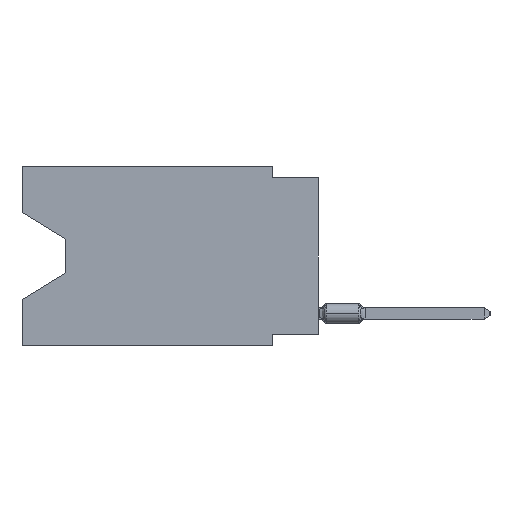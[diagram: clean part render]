
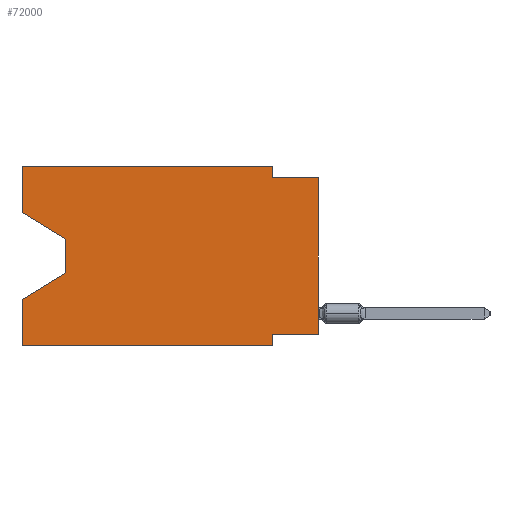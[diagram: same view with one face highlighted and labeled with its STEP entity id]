
A CAD part, left-side view. The second image highlights one B-rep face of the part: STEP entity #72000.
In plain terms, the highlighted planar face has unit normal (-1, 0, 0).
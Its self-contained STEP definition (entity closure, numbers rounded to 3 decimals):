
#440 = CARTESIAN_POINT ( 'NONE',  ( 0., 16.383, 0. ) ) ;
#507 = CARTESIAN_POINT ( 'NONE',  ( 0., 16.383, 0. ) ) ;
#642 = CARTESIAN_POINT ( 'NONE',  ( 0., 2.54, -9.906 ) ) ;
#739 = EDGE_CURVE ( 'NONE', #52487, #64820, #70216, .T. ) ;
#3649 = DIRECTION ( 'NONE',  ( 0., -1., 0. ) ) ;
#3943 = EDGE_LOOP ( 'NONE', ( #4611, #56221, #51266, #8368, #60722, #46867, #68216, #13550, #81424, #51100, #72650, #27311 ) ) ;
#4611 = ORIENTED_EDGE ( 'NONE', *, *, #12459, .T. ) ;
#5242 = CARTESIAN_POINT ( 'NONE',  ( 0., 16.383, -9.906 ) ) ;
#6098 = CARTESIAN_POINT ( 'NONE',  ( 0., 0., -9.271 ) ) ;
#8295 = EDGE_CURVE ( 'NONE', #15607, #71656, #63354, .T. ) ;
#8368 = ORIENTED_EDGE ( 'NONE', *, *, #38040, .F. ) ;
#9040 = DIRECTION ( 'NONE',  ( 0., 0., -1. ) ) ;
#9926 = CARTESIAN_POINT ( 'NONE',  ( 0., 0., -0.635 ) ) ;
#12459 = EDGE_CURVE ( 'NONE', #52487, #46699, #63314, .T. ) ;
#12963 = CARTESIAN_POINT ( 'NONE',  ( 0., 16.383, 0. ) ) ;
#13550 = ORIENTED_EDGE ( 'NONE', *, *, #52747, .T. ) ;
#13560 = DIRECTION ( 'NONE',  ( 0., -0.855, -0.519 ) ) ;
#15607 = VERTEX_POINT ( 'NONE', #53150 ) ;
#16781 = DIRECTION ( 'NONE',  ( 0., 0., -1. ) ) ;
#18680 = LINE ( 'NONE', #26591, #46604 ) ;
#19165 = VERTEX_POINT ( 'NONE', #642 ) ;
#20606 = LINE ( 'NONE', #39845, #56471 ) ;
#21585 = FACE_OUTER_BOUND ( 'NONE', #3943, .T. ) ;
#22168 = VECTOR ( 'NONE', #16781, 1000. ) ;
#22882 = EDGE_CURVE ( 'NONE', #46699, #24550, #68189, .T. ) ;
#23731 = CARTESIAN_POINT ( 'NONE',  ( 0., 16.383, -2.546 ) ) ;
#24550 = VERTEX_POINT ( 'NONE', #35504 ) ;
#24556 = DIRECTION ( 'NONE',  ( 0., 0.855, -0.519 ) ) ;
#24721 = VERTEX_POINT ( 'NONE', #5242 ) ;
#25302 = LINE ( 'NONE', #73493, #69321 ) ;
#25745 = VERTEX_POINT ( 'NONE', #40839 ) ;
#26591 = CARTESIAN_POINT ( 'NONE',  ( 0., 0., 0. ) ) ;
#27300 = DIRECTION ( 'NONE',  ( 0., 0., -1. ) ) ;
#27311 = ORIENTED_EDGE ( 'NONE', *, *, #739, .F. ) ;
#28710 = EDGE_CURVE ( 'NONE', #64820, #25745, #45646, .T. ) ;
#29109 = PLANE ( 'NONE',  #66362 ) ;
#29790 = EDGE_CURVE ( 'NONE', #25745, #72298, #55531, .T. ) ;
#30439 = LINE ( 'NONE', #36698, #69041 ) ;
#31791 = DIRECTION ( 'NONE',  ( 0., 0., 1. ) ) ;
#32022 = DIRECTION ( 'NONE',  ( 0., 1., 0. ) ) ;
#34330 = CARTESIAN_POINT ( 'NONE',  ( 0., 2.54, -9.271 ) ) ;
#34546 = CARTESIAN_POINT ( 'NONE',  ( 0., 16.383, 0. ) ) ;
#35504 = CARTESIAN_POINT ( 'NONE',  ( 0., 13.97, -5.893 ) ) ;
#35910 = CARTESIAN_POINT ( 'NONE',  ( 0., 2.54, 0. ) ) ;
#36677 = LINE ( 'NONE', #9926, #48466 ) ;
#36698 = CARTESIAN_POINT ( 'NONE',  ( 0., 13.97, -5.893 ) ) ;
#38040 = EDGE_CURVE ( 'NONE', #24721, #42296, #25302, .T. ) ;
#38560 = DIRECTION ( 'NONE',  ( 0., -1., 0. ) ) ;
#39845 = CARTESIAN_POINT ( 'NONE',  ( 0., 16.383, -9.906 ) ) ;
#40214 = EDGE_CURVE ( 'NONE', #24550, #42296, #30439, .T. ) ;
#40839 = CARTESIAN_POINT ( 'NONE',  ( 0., 2.54, 0. ) ) ;
#42296 = VERTEX_POINT ( 'NONE', #53952 ) ;
#42703 = CARTESIAN_POINT ( 'NONE',  ( 0., 13.97, -4.013 ) ) ;
#43005 = DIRECTION ( 'NONE',  ( 0., 0., -1. ) ) ;
#44108 = CARTESIAN_POINT ( 'NONE',  ( 0., 16.383, -2.546 ) ) ;
#45646 = LINE ( 'NONE', #507, #59222 ) ;
#46604 = VECTOR ( 'NONE', #52079, 1000. ) ;
#46699 = VERTEX_POINT ( 'NONE', #47938 ) ;
#46867 = ORIENTED_EDGE ( 'NONE', *, *, #68709, .F. ) ;
#47938 = CARTESIAN_POINT ( 'NONE',  ( 0., 13.97, -4.013 ) ) ;
#48466 = VECTOR ( 'NONE', #3649, 1000. ) ;
#51100 = ORIENTED_EDGE ( 'NONE', *, *, #29790, .F. ) ;
#51266 = ORIENTED_EDGE ( 'NONE', *, *, #40214, .T. ) ;
#52079 = DIRECTION ( 'NONE',  ( 0., 0., 1. ) ) ;
#52487 = VERTEX_POINT ( 'NONE', #23731 ) ;
#52747 = EDGE_CURVE ( 'NONE', #15607, #66571, #18680, .T. ) ;
#52821 = VECTOR ( 'NONE', #27300, 1000. ) ;
#53150 = CARTESIAN_POINT ( 'NONE',  ( 0., 0., -9.271 ) ) ;
#53952 = CARTESIAN_POINT ( 'NONE',  ( 0., 16.383, -7.36 ) ) ;
#55531 = LINE ( 'NONE', #35910, #78062 ) ;
#56221 = ORIENTED_EDGE ( 'NONE', *, *, #22882, .T. ) ;
#56471 = VECTOR ( 'NONE', #58638, 1000. ) ;
#56646 = EDGE_CURVE ( 'NONE', #72298, #66571, #36677, .T. ) ;
#58638 = DIRECTION ( 'NONE',  ( 0., -1., 0. ) ) ;
#59222 = VECTOR ( 'NONE', #38560, 1000. ) ;
#59672 = CARTESIAN_POINT ( 'NONE',  ( 0., 0., -0.635 ) ) ;
#59866 = CARTESIAN_POINT ( 'NONE',  ( 0., 2.54, -9.906 ) ) ;
#60722 = ORIENTED_EDGE ( 'NONE', *, *, #65756, .T. ) ;
#63314 = LINE ( 'NONE', #44108, #67693 ) ;
#63354 = LINE ( 'NONE', #6098, #79180 ) ;
#63713 = CARTESIAN_POINT ( 'NONE',  ( 0., 2.54, -0.635 ) ) ;
#64820 = VERTEX_POINT ( 'NONE', #440 ) ;
#65738 = LINE ( 'NONE', #59866, #52821 ) ;
#65756 = EDGE_CURVE ( 'NONE', #24721, #19165, #20606, .T. ) ;
#66362 = AXIS2_PLACEMENT_3D ( 'NONE', #34546, #77978, #9040 ) ;
#66424 = VECTOR ( 'NONE', #31791, 1000. ) ;
#66571 = VERTEX_POINT ( 'NONE', #59672 ) ;
#67693 = VECTOR ( 'NONE', #13560, 1000. ) ;
#68189 = LINE ( 'NONE', #42703, #22168 ) ;
#68216 = ORIENTED_EDGE ( 'NONE', *, *, #8295, .F. ) ;
#68709 = EDGE_CURVE ( 'NONE', #71656, #19165, #65738, .T. ) ;
#69041 = VECTOR ( 'NONE', #24556, 1000. ) ;
#69321 = VECTOR ( 'NONE', #80572, 1000. ) ;
#70216 = LINE ( 'NONE', #12963, #66424 ) ;
#71656 = VERTEX_POINT ( 'NONE', #34330 ) ;
#72000 = ADVANCED_FACE ( 'NONE', ( #21585 ), #29109, .F. ) ;
#72298 = VERTEX_POINT ( 'NONE', #63713 ) ;
#72650 = ORIENTED_EDGE ( 'NONE', *, *, #28710, .F. ) ;
#73493 = CARTESIAN_POINT ( 'NONE',  ( 0., 16.383, 0. ) ) ;
#77978 = DIRECTION ( 'NONE',  ( 1., 0., 0. ) ) ;
#78062 = VECTOR ( 'NONE', #43005, 1000. ) ;
#79180 = VECTOR ( 'NONE', #32022, 1000. ) ;
#80572 = DIRECTION ( 'NONE',  ( 0., 0., 1. ) ) ;
#81424 = ORIENTED_EDGE ( 'NONE', *, *, #56646, .F. ) ;
